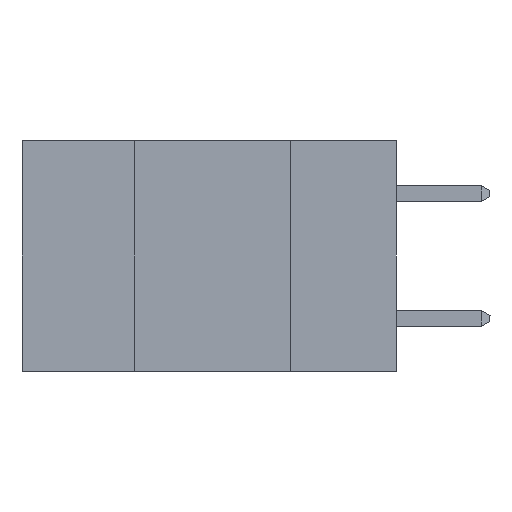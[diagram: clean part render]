
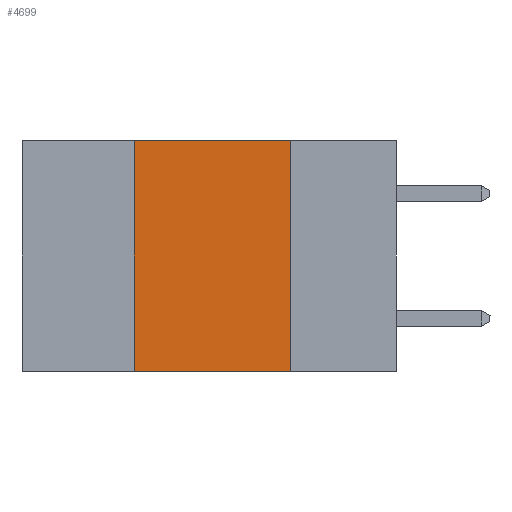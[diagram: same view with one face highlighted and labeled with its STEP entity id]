
A CAD part, left-side view. The second image highlights one B-rep face of the part: STEP entity #4699.
In plain terms, the highlighted planar face has unit normal (-1, 0, 0).
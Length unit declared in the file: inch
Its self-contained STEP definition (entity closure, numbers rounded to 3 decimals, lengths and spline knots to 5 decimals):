
#447 = DIRECTION ( 'NONE',  ( 0., -1., 0. ) ) ;
#1134 = EDGE_CURVE ( 'NONE', #2300, #4185, #5959, .T. ) ;
#1760 = DIRECTION ( 'NONE',  ( 1., 0., 0. ) ) ;
#2032 = ORIENTED_EDGE ( 'NONE', *, *, #8707, .F. ) ;
#2300 = VERTEX_POINT ( 'NONE', #13075 ) ;
#2340 = LINE ( 'NONE', #12920, #11667 ) ;
#2782 = ORIENTED_EDGE ( 'NONE', *, *, #9985, .F. ) ;
#3648 = VECTOR ( 'NONE', #447, 39.37008 ) ;
#4185 = VERTEX_POINT ( 'NONE', #7266 ) ;
#4699 = ADVANCED_FACE ( 'NONE', ( #15126 ), #13182, .F. ) ;
#4782 = CARTESIAN_POINT ( 'NONE',  ( 0., 0.17, 0. ) ) ;
#5383 = DIRECTION ( 'NONE',  ( 0., 0., 1. ) ) ;
#5558 = VERTEX_POINT ( 'NONE', #12251 ) ;
#5959 = LINE ( 'NONE', #6310, #8966 ) ;
#6310 = CARTESIAN_POINT ( 'NONE',  ( 0., 0.6, -0.37 ) ) ;
#7156 = VECTOR ( 'NONE', #13187, 39.37008 ) ;
#7266 = CARTESIAN_POINT ( 'NONE',  ( 0., 0.17, -0.37 ) ) ;
#7972 = ORIENTED_EDGE ( 'NONE', *, *, #1134, .T. ) ;
#8707 = EDGE_CURVE ( 'NONE', #14439, #4185, #10543, .T. ) ;
#8966 = VECTOR ( 'NONE', #11203, 39.37008 ) ;
#9985 = EDGE_CURVE ( 'NONE', #2300, #5558, #2340, .T. ) ;
#10422 = LINE ( 'NONE', #15607, #3648 ) ;
#10543 = LINE ( 'NONE', #15639, #7156 ) ;
#11203 = DIRECTION ( 'NONE',  ( 0., -1., 0. ) ) ;
#11667 = VECTOR ( 'NONE', #5383, 39.37008 ) ;
#11906 = CARTESIAN_POINT ( 'NONE',  ( 0., 0.6, 0. ) ) ;
#11977 = EDGE_CURVE ( 'NONE', #5558, #14439, #10422, .T. ) ;
#12251 = CARTESIAN_POINT ( 'NONE',  ( 0., 0.42, 0. ) ) ;
#12920 = CARTESIAN_POINT ( 'NONE',  ( 0., 0.42, -0.37 ) ) ;
#13075 = CARTESIAN_POINT ( 'NONE',  ( 0., 0.42, -0.37 ) ) ;
#13182 = PLANE ( 'NONE',  #15597 ) ;
#13187 = DIRECTION ( 'NONE',  ( 0., 0., -1. ) ) ;
#14439 = VERTEX_POINT ( 'NONE', #4782 ) ;
#14448 = DIRECTION ( 'NONE',  ( 0., 0., -1. ) ) ;
#15126 = FACE_OUTER_BOUND ( 'NONE', #15515, .T. ) ;
#15515 = EDGE_LOOP ( 'NONE', ( #2032, #16262, #2782, #7972 ) ) ;
#15597 = AXIS2_PLACEMENT_3D ( 'NONE', #11906, #1760, #14448 ) ;
#15607 = CARTESIAN_POINT ( 'NONE',  ( 0., 0.6, 0. ) ) ;
#15639 = CARTESIAN_POINT ( 'NONE',  ( 0., 0.17, -0.37 ) ) ;
#16262 = ORIENTED_EDGE ( 'NONE', *, *, #11977, .F. ) ;
